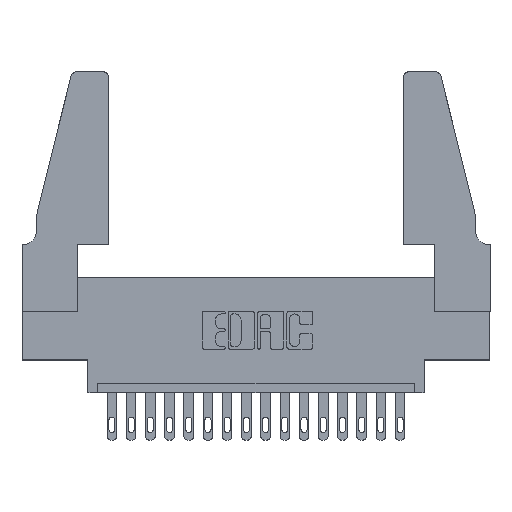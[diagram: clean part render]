
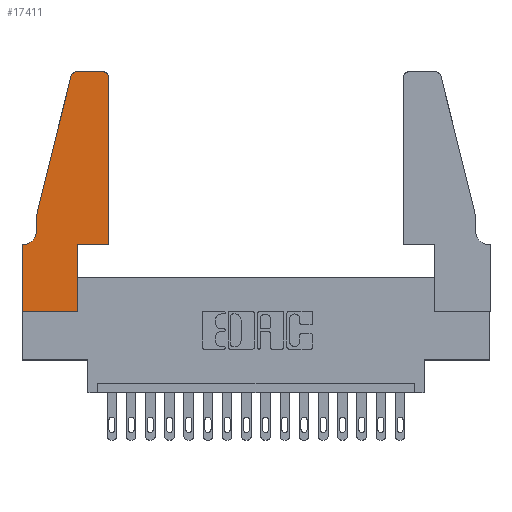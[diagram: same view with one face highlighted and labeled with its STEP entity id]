
A CAD part, top view. The second image highlights one B-rep face of the part: STEP entity #17411.
In plain terms, the highlighted planar face has unit normal (0, 0, 1).
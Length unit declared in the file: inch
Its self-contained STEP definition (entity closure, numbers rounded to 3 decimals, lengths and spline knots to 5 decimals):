
#25 = EDGE_CURVE ( 'NONE', #9042, #4287, #10051, .T. ) ;
#96 = VECTOR ( 'NONE', #10858, 39.37008 ) ;
#102 = VECTOR ( 'NONE', #2082, 39.37008 ) ;
#335 = VERTEX_POINT ( 'NONE', #5365 ) ;
#349 = EDGE_CURVE ( 'NONE', #13003, #15360, #11291, .T. ) ;
#383 = VECTOR ( 'NONE', #2253, 39.37008 ) ;
#535 = DIRECTION ( 'NONE',  ( -1., 0., 0. ) ) ;
#625 = CARTESIAN_POINT ( 'NONE',  ( 0.2865, 0.35, 0.37 ) ) ;
#692 = ORIENTED_EDGE ( 'NONE', *, *, #16064, .T. ) ;
#784 = ORIENTED_EDGE ( 'NONE', *, *, #14440, .T. ) ;
#973 = CARTESIAN_POINT ( 'NONE',  ( 0., 0., 0.37 ) ) ;
#1090 = CARTESIAN_POINT ( 'NONE',  ( 0.4205, 1.22, 0.37 ) ) ;
#1150 = ORIENTED_EDGE ( 'NONE', *, *, #11087, .T. ) ;
#1257 = CARTESIAN_POINT ( 'NONE',  ( 0.25487, 1.22718, 0.37 ) ) ;
#1595 = LINE ( 'NONE', #6105, #102 ) ;
#1666 = VERTEX_POINT ( 'NONE', #1257 ) ;
#1730 = CARTESIAN_POINT ( 'NONE',  ( 0.0055, 0.42, 0.37 ) ) ;
#1794 = ORIENTED_EDGE ( 'NONE', *, *, #6256, .T. ) ;
#1817 = FACE_OUTER_BOUND ( 'NONE', #15515, .T. ) ;
#2082 = DIRECTION ( 'NONE',  ( 0., -1., 0. ) ) ;
#2084 = LINE ( 'NONE', #9496, #12135 ) ;
#2188 = CIRCLE ( 'NONE', #6734, 0.03 ) ;
#2239 = VERTEX_POINT ( 'NONE', #973 ) ;
#2253 = DIRECTION ( 'NONE',  ( 0., 1., 0. ) ) ;
#2382 = ORIENTED_EDGE ( 'NONE', *, *, #10198, .T. ) ;
#2402 = DIRECTION ( 'NONE',  ( 1., 0., 0. ) ) ;
#2455 = DIRECTION ( 'NONE',  ( 0., 0., 1. ) ) ;
#2545 = LINE ( 'NONE', #9045, #383 ) ;
#2600 = VECTOR ( 'NONE', #8082, 39.37008 ) ;
#2671 = LINE ( 'NONE', #12140, #96 ) ;
#2698 = CARTESIAN_POINT ( 'NONE',  ( 0.4505, 0.35, 0.37 ) ) ;
#2809 = AXIS2_PLACEMENT_3D ( 'NONE', #1090, #2455, #17559 ) ;
#2948 = CARTESIAN_POINT ( 'NONE',  ( 0.284, 1.25, 0.37 ) ) ;
#3002 = EDGE_CURVE ( 'NONE', #15360, #1666, #2188, .T. ) ;
#3411 = LINE ( 'NONE', #12829, #13467 ) ;
#4287 = VERTEX_POINT ( 'NONE', #625 ) ;
#5365 = CARTESIAN_POINT ( 'NONE',  ( 0.0055, 0.35, 0.37 ) ) ;
#5862 = ORIENTED_EDGE ( 'NONE', *, *, #14261, .T. ) ;
#6105 = CARTESIAN_POINT ( 'NONE',  ( 0.0755, 0.5, 0.37 ) ) ;
#6256 = EDGE_CURVE ( 'NONE', #8501, #15741, #2545, .T. ) ;
#6734 = AXIS2_PLACEMENT_3D ( 'NONE', #12130, #10952, #9553 ) ;
#7398 = AXIS2_PLACEMENT_3D ( 'NONE', #16534, #16359, #15037 ) ;
#7799 = CIRCLE ( 'NONE', #12624, 0.07 ) ;
#8050 = CARTESIAN_POINT ( 'NONE',  ( 0.2865, 0., 0.37 ) ) ;
#8082 = DIRECTION ( 'NONE',  ( -1., 0., 0. ) ) ;
#8335 = EDGE_CURVE ( 'NONE', #1666, #13611, #2671, .T. ) ;
#8501 = VERTEX_POINT ( 'NONE', #2698 ) ;
#9039 = ORIENTED_EDGE ( 'NONE', *, *, #3002, .T. ) ;
#9042 = VERTEX_POINT ( 'NONE', #8050 ) ;
#9045 = CARTESIAN_POINT ( 'NONE',  ( 0.4505, 0.35, 0.37 ) ) ;
#9496 = CARTESIAN_POINT ( 'NONE',  ( 0., 0., 0.37 ) ) ;
#9553 = DIRECTION ( 'NONE',  ( 1., 0., 0. ) ) ;
#9660 = CARTESIAN_POINT ( 'NONE',  ( 0.2865, 0.35, 0.37 ) ) ;
#9791 = VERTEX_POINT ( 'NONE', #14808 ) ;
#10022 = VECTOR ( 'NONE', #15351, 39.37008 ) ;
#10051 = LINE ( 'NONE', #9660, #15233 ) ;
#10198 = EDGE_CURVE ( 'NONE', #15741, #13003, #11992, .T. ) ;
#10225 = VERTEX_POINT ( 'NONE', #17617 ) ;
#10479 = CARTESIAN_POINT ( 'NONE',  ( 0.4505, 0.35, 0.37 ) ) ;
#10784 = PLANE ( 'NONE',  #7398 ) ;
#10858 = DIRECTION ( 'NONE',  ( -0.239, -0.971, 0. ) ) ;
#10952 = DIRECTION ( 'NONE',  ( 0., 0., 1. ) ) ;
#11004 = DIRECTION ( 'NONE',  ( 0., 1., 0. ) ) ;
#11087 = EDGE_CURVE ( 'NONE', #4287, #8501, #16516, .T. ) ;
#11218 = EDGE_CURVE ( 'NONE', #335, #9791, #3411, .T. ) ;
#11261 = CARTESIAN_POINT ( 'NONE',  ( 0., 0., 0.37 ) ) ;
#11291 = LINE ( 'NONE', #17573, #2600 ) ;
#11482 = ORIENTED_EDGE ( 'NONE', *, *, #349, .T. ) ;
#11992 = CIRCLE ( 'NONE', #2809, 0.03 ) ;
#12017 = EDGE_CURVE ( 'NONE', #2239, #9042, #2084, .T. ) ;
#12130 = CARTESIAN_POINT ( 'NONE',  ( 0.284, 1.22, 0.37 ) ) ;
#12135 = VECTOR ( 'NONE', #2402, 39.37008 ) ;
#12140 = CARTESIAN_POINT ( 'NONE',  ( 0.0755, 0.5, 0.37 ) ) ;
#12624 = AXIS2_PLACEMENT_3D ( 'NONE', #1730, #15458, #12781 ) ;
#12781 = DIRECTION ( 'NONE',  ( -1., 0., 0. ) ) ;
#12792 = CARTESIAN_POINT ( 'NONE',  ( 0.4505, 1.22, 0.37 ) ) ;
#12829 = CARTESIAN_POINT ( 'NONE',  ( 0.0755, 0.35, 0.37 ) ) ;
#13003 = VERTEX_POINT ( 'NONE', #16744 ) ;
#13467 = VECTOR ( 'NONE', #535, 39.37008 ) ;
#13611 = VERTEX_POINT ( 'NONE', #14274 ) ;
#13918 = ORIENTED_EDGE ( 'NONE', *, *, #11218, .T. ) ;
#14261 = EDGE_CURVE ( 'NONE', #10225, #335, #7799, .T. ) ;
#14274 = CARTESIAN_POINT ( 'NONE',  ( 0.0755, 0.5, 0.37 ) ) ;
#14440 = EDGE_CURVE ( 'NONE', #13611, #10225, #1595, .T. ) ;
#14808 = CARTESIAN_POINT ( 'NONE',  ( 0., 0.35, 0.37 ) ) ;
#15037 = DIRECTION ( 'NONE',  ( 1., 0., 0. ) ) ;
#15160 = ORIENTED_EDGE ( 'NONE', *, *, #12017, .T. ) ;
#15233 = VECTOR ( 'NONE', #11004, 39.37008 ) ;
#15351 = DIRECTION ( 'NONE',  ( 1., 0., 0. ) ) ;
#15360 = VERTEX_POINT ( 'NONE', #2948 ) ;
#15417 = DIRECTION ( 'NONE',  ( 0., -1., 0. ) ) ;
#15458 = DIRECTION ( 'NONE',  ( 0., 0., -1. ) ) ;
#15515 = EDGE_LOOP ( 'NONE', ( #11482, #9039, #17779, #784, #5862, #13918, #692, #15160, #16775, #1150, #1794, #2382 ) ) ;
#15741 = VERTEX_POINT ( 'NONE', #12792 ) ;
#16064 = EDGE_CURVE ( 'NONE', #9791, #2239, #16685, .T. ) ;
#16359 = DIRECTION ( 'NONE',  ( 0., 0., 1. ) ) ;
#16516 = LINE ( 'NONE', #10479, #10022 ) ;
#16534 = CARTESIAN_POINT ( 'NONE',  ( 0., 0.35, 0.37 ) ) ;
#16685 = LINE ( 'NONE', #11261, #17099 ) ;
#16744 = CARTESIAN_POINT ( 'NONE',  ( 0.4205, 1.25, 0.37 ) ) ;
#16775 = ORIENTED_EDGE ( 'NONE', *, *, #25, .T. ) ;
#17099 = VECTOR ( 'NONE', #15417, 39.37008 ) ;
#17411 = ADVANCED_FACE ( 'NONE', ( #1817 ), #10784, .T. ) ;
#17559 = DIRECTION ( 'NONE',  ( 1., 0., 0. ) ) ;
#17573 = CARTESIAN_POINT ( 'NONE',  ( 0.2605, 1.25, 0.37 ) ) ;
#17617 = CARTESIAN_POINT ( 'NONE',  ( 0.0755, 0.42, 0.37 ) ) ;
#17779 = ORIENTED_EDGE ( 'NONE', *, *, #8335, .T. ) ;
